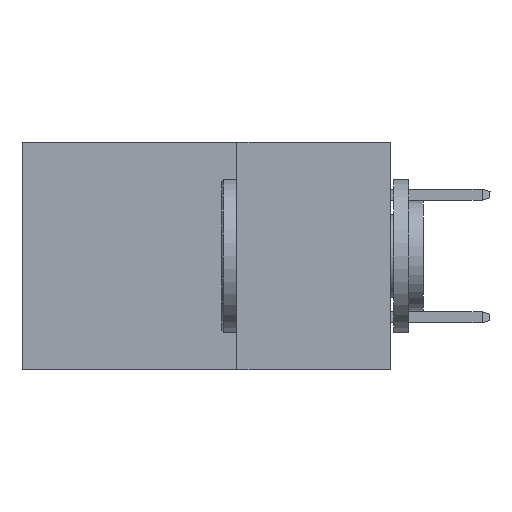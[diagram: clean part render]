
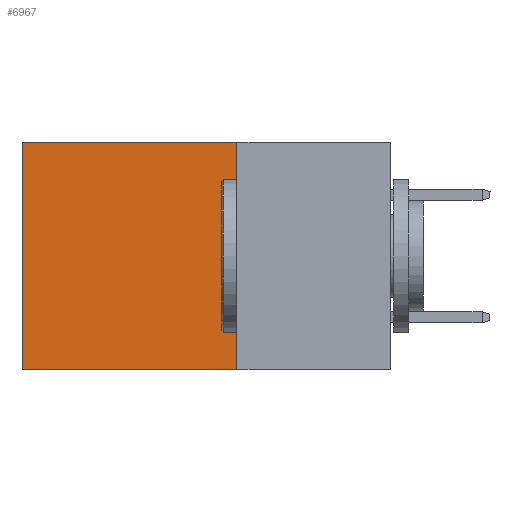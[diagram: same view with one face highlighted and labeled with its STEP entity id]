
A CAD part, left-side view. The second image highlights one B-rep face of the part: STEP entity #6967.
In plain terms, the highlighted planar face has unit normal (-1, 0, 0).
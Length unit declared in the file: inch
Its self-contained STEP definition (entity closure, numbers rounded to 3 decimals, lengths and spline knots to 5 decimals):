
#147 = DIRECTION ( 'NONE',  ( 0., 0., -1. ) ) ;
#451 = LINE ( 'NONE', #6019, #3819 ) ;
#537 = ORIENTED_EDGE ( 'NONE', *, *, #12939, .F. ) ;
#666 = ORIENTED_EDGE ( 'NONE', *, *, #6652, .T. ) ;
#1394 = CARTESIAN_POINT ( 'NONE',  ( 0.2875, 0.6, 0. ) ) ;
#1788 = AXIS2_PLACEMENT_3D ( 'NONE', #16548, #11428, #3181 ) ;
#1814 = PLANE ( 'NONE',  #1788 ) ;
#1903 = ORIENTED_EDGE ( 'NONE', *, *, #6944, .T. ) ;
#3181 = DIRECTION ( 'NONE',  ( 0., 0., -1. ) ) ;
#3819 = VECTOR ( 'NONE', #5945, 39.37008 ) ;
#4250 = CARTESIAN_POINT ( 'NONE',  ( 0.2875, 0.25, 0. ) ) ;
#5945 = DIRECTION ( 'NONE',  ( 0., 1., 0. ) ) ;
#6019 = CARTESIAN_POINT ( 'NONE',  ( 0.2875, 0.25, -0.37 ) ) ;
#6652 = EDGE_CURVE ( 'NONE', #9898, #7142, #7521, .T. ) ;
#6944 = EDGE_CURVE ( 'NONE', #7142, #19955, #14697, .T. ) ;
#6967 = ADVANCED_FACE ( 'NONE', ( #19115 ), #1814, .F. ) ;
#7133 = CARTESIAN_POINT ( 'NONE',  ( 0.2875, 0.6, -0.37 ) ) ;
#7141 = DIRECTION ( 'NONE',  ( 0., 1., 0. ) ) ;
#7142 = VERTEX_POINT ( 'NONE', #16903 ) ;
#7521 = LINE ( 'NONE', #8713, #13444 ) ;
#7693 = CARTESIAN_POINT ( 'NONE',  ( 0.2875, 0.25, -0.37 ) ) ;
#8388 = VECTOR ( 'NONE', #17211, 39.37008 ) ;
#8713 = CARTESIAN_POINT ( 'NONE',  ( 0.2875, 0.25, 0. ) ) ;
#9898 = VERTEX_POINT ( 'NONE', #4250 ) ;
#10080 = VECTOR ( 'NONE', #147, 39.37008 ) ;
#10171 = ORIENTED_EDGE ( 'NONE', *, *, #20240, .F. ) ;
#10357 = EDGE_LOOP ( 'NONE', ( #1903, #537, #10171, #666 ) ) ;
#10505 = CARTESIAN_POINT ( 'NONE',  ( 0.2875, 0.25, 0. ) ) ;
#11428 = DIRECTION ( 'NONE',  ( 1., 0., 0. ) ) ;
#12760 = LINE ( 'NONE', #10505, #8388 ) ;
#12939 = EDGE_CURVE ( 'NONE', #16051, #19955, #451, .T. ) ;
#13444 = VECTOR ( 'NONE', #7141, 39.37008 ) ;
#14697 = LINE ( 'NONE', #1394, #10080 ) ;
#16051 = VERTEX_POINT ( 'NONE', #7693 ) ;
#16548 = CARTESIAN_POINT ( 'NONE',  ( 0.2875, 0.25, 0. ) ) ;
#16903 = CARTESIAN_POINT ( 'NONE',  ( 0.2875, 0.6, 0. ) ) ;
#17211 = DIRECTION ( 'NONE',  ( 0., 0., -1. ) ) ;
#19115 = FACE_OUTER_BOUND ( 'NONE', #10357, .T. ) ;
#19955 = VERTEX_POINT ( 'NONE', #7133 ) ;
#20240 = EDGE_CURVE ( 'NONE', #9898, #16051, #12760, .T. ) ;
